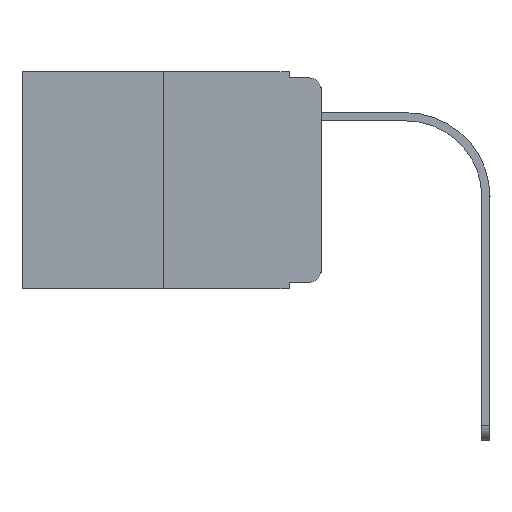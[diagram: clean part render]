
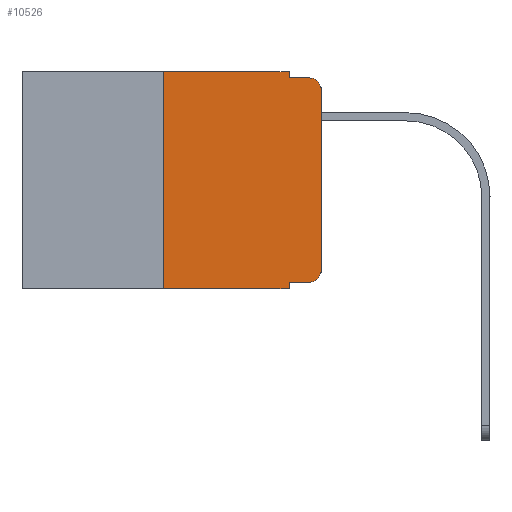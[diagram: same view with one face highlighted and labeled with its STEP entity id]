
A CAD part, left-side view. The second image highlights one B-rep face of the part: STEP entity #10526.
In plain terms, the highlighted planar face has unit normal (-1, 0, 0).
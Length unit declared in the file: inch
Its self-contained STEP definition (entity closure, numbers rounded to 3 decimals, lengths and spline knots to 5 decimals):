
#642 = ORIENTED_EDGE ( 'NONE', *, *, #10785, .F. ) ;
#699 = VERTEX_POINT ( 'NONE', #12797 ) ;
#761 = ORIENTED_EDGE ( 'NONE', *, *, #13675, .T. ) ;
#852 = LINE ( 'NONE', #12098, #2911 ) ;
#1095 = DIRECTION ( 'NONE',  ( 0., 0., -1. ) ) ;
#1178 = DIRECTION ( 'NONE',  ( 1., 0., 0. ) ) ;
#1365 = VERTEX_POINT ( 'NONE', #4801 ) ;
#1489 = DIRECTION ( 'NONE',  ( -1., 0., 0. ) ) ;
#1663 = VECTOR ( 'NONE', #3210, 39.37008 ) ;
#1671 = ORIENTED_EDGE ( 'NONE', *, *, #2084, .F. ) ;
#1684 = DIRECTION ( 'NONE',  ( -1., 0., 0. ) ) ;
#1687 = VECTOR ( 'NONE', #1709, 39.37008 ) ;
#1709 = DIRECTION ( 'NONE',  ( 0., -1., 0. ) ) ;
#1920 = CARTESIAN_POINT ( 'NONE',  ( 0., 0.051, -0.333 ) ) ;
#1997 = CARTESIAN_POINT ( 'NONE',  ( 0., 0.02, -0.333 ) ) ;
#2084 = EDGE_CURVE ( 'NONE', #699, #5482, #10360, .T. ) ;
#2117 = VECTOR ( 'NONE', #14281, 39.37008 ) ;
#2717 = LINE ( 'NONE', #15356, #7923 ) ;
#2911 = VECTOR ( 'NONE', #8301, 39.37008 ) ;
#3184 = VECTOR ( 'NONE', #4369, 39.37008 ) ;
#3191 = EDGE_CURVE ( 'NONE', #8622, #5011, #15493, .T. ) ;
#3210 = DIRECTION ( 'NONE',  ( 0., -1., 0. ) ) ;
#3257 = ORIENTED_EDGE ( 'NONE', *, *, #3451, .F. ) ;
#3451 = EDGE_CURVE ( 'NONE', #8622, #6676, #2717, .T. ) ;
#3988 = AXIS2_PLACEMENT_3D ( 'NONE', #4334, #1684, #9280 ) ;
#4334 = CARTESIAN_POINT ( 'NONE',  ( 0., 0.02, -0.03 ) ) ;
#4351 = EDGE_CURVE ( 'NONE', #5482, #6927, #13937, .T. ) ;
#4356 = CARTESIAN_POINT ( 'NONE',  ( 0., 0., -0.03 ) ) ;
#4369 = DIRECTION ( 'NONE',  ( 0., 0., -1. ) ) ;
#4468 = ORIENTED_EDGE ( 'NONE', *, *, #3191, .T. ) ;
#4512 = EDGE_CURVE ( 'NONE', #13848, #5011, #5578, .T. ) ;
#4595 = CARTESIAN_POINT ( 'NONE',  ( 0., 0.25, -0.343 ) ) ;
#4801 = CARTESIAN_POINT ( 'NONE',  ( 0., 0., -0.313 ) ) ;
#5011 = VERTEX_POINT ( 'NONE', #14778 ) ;
#5345 = CARTESIAN_POINT ( 'NONE',  ( 0., 0.25, 0. ) ) ;
#5482 = VERTEX_POINT ( 'NONE', #10277 ) ;
#5578 = LINE ( 'NONE', #9300, #10788 ) ;
#5629 = LINE ( 'NONE', #1920, #1663 ) ;
#5694 = CARTESIAN_POINT ( 'NONE',  ( 0., 0.473, 0. ) ) ;
#6269 = PLANE ( 'NONE',  #9319 ) ;
#6667 = DIRECTION ( 'NONE',  ( 0., 0., 1. ) ) ;
#6676 = VERTEX_POINT ( 'NONE', #5345 ) ;
#6927 = VERTEX_POINT ( 'NONE', #15793 ) ;
#7727 = CIRCLE ( 'NONE', #10307, 0.02 ) ;
#7923 = VECTOR ( 'NONE', #6667, 39.37008 ) ;
#8301 = DIRECTION ( 'NONE',  ( 0., 0., 1. ) ) ;
#8622 = VERTEX_POINT ( 'NONE', #4595 ) ;
#8678 = VERTEX_POINT ( 'NONE', #4356 ) ;
#8835 = CARTESIAN_POINT ( 'NONE',  ( 0., 0.051, -0.01 ) ) ;
#8904 = CIRCLE ( 'NONE', #3988, 0.02 ) ;
#9280 = DIRECTION ( 'NONE',  ( 0., 0., -1. ) ) ;
#9300 = CARTESIAN_POINT ( 'NONE',  ( 0., 0.051, 0. ) ) ;
#9319 = AXIS2_PLACEMENT_3D ( 'NONE', #16005, #1178, #1095 ) ;
#9321 = CARTESIAN_POINT ( 'NONE',  ( 0., 0.473, -0.343 ) ) ;
#9841 = VECTOR ( 'NONE', #15437, 39.37008 ) ;
#10277 = CARTESIAN_POINT ( 'NONE',  ( 0., 0.051, -0.01 ) ) ;
#10307 = AXIS2_PLACEMENT_3D ( 'NONE', #12580, #1489, #14788 ) ;
#10360 = LINE ( 'NONE', #15482, #3184 ) ;
#10417 = VERTEX_POINT ( 'NONE', #1997 ) ;
#10526 = ADVANCED_FACE ( 'NONE', ( #11037 ), #6269, .F. ) ;
#10567 = EDGE_LOOP ( 'NONE', ( #11794, #761, #13533, #1671, #642, #3257, #4468, #12792, #12236, #14541 ) ) ;
#10785 = EDGE_CURVE ( 'NONE', #6676, #699, #12900, .T. ) ;
#10788 = VECTOR ( 'NONE', #11646, 39.37008 ) ;
#11037 = FACE_OUTER_BOUND ( 'NONE', #10567, .T. ) ;
#11646 = DIRECTION ( 'NONE',  ( 0., 0., -1. ) ) ;
#11794 = ORIENTED_EDGE ( 'NONE', *, *, #12463, .T. ) ;
#12098 = CARTESIAN_POINT ( 'NONE',  ( 0., 0., 0. ) ) ;
#12236 = ORIENTED_EDGE ( 'NONE', *, *, #13638, .T. ) ;
#12463 = EDGE_CURVE ( 'NONE', #1365, #8678, #852, .T. ) ;
#12580 = CARTESIAN_POINT ( 'NONE',  ( 0., 0.02, -0.313 ) ) ;
#12792 = ORIENTED_EDGE ( 'NONE', *, *, #4512, .F. ) ;
#12797 = CARTESIAN_POINT ( 'NONE',  ( 0., 0.051, 0. ) ) ;
#12900 = LINE ( 'NONE', #5694, #9841 ) ;
#13533 = ORIENTED_EDGE ( 'NONE', *, *, #4351, .F. ) ;
#13638 = EDGE_CURVE ( 'NONE', #13848, #10417, #5629, .T. ) ;
#13675 = EDGE_CURVE ( 'NONE', #8678, #6927, #8904, .T. ) ;
#13848 = VERTEX_POINT ( 'NONE', #16002 ) ;
#13937 = LINE ( 'NONE', #8835, #1687 ) ;
#14281 = DIRECTION ( 'NONE',  ( 0., -1., 0. ) ) ;
#14541 = ORIENTED_EDGE ( 'NONE', *, *, #15978, .T. ) ;
#14778 = CARTESIAN_POINT ( 'NONE',  ( 0., 0.051, -0.343 ) ) ;
#14788 = DIRECTION ( 'NONE',  ( 0., 0., -1. ) ) ;
#15356 = CARTESIAN_POINT ( 'NONE',  ( 0., 0.25, 0. ) ) ;
#15437 = DIRECTION ( 'NONE',  ( 0., -1., 0. ) ) ;
#15482 = CARTESIAN_POINT ( 'NONE',  ( 0., 0.051, 0. ) ) ;
#15493 = LINE ( 'NONE', #9321, #2117 ) ;
#15793 = CARTESIAN_POINT ( 'NONE',  ( 0., 0.02, -0.01 ) ) ;
#15978 = EDGE_CURVE ( 'NONE', #10417, #1365, #7727, .T. ) ;
#16002 = CARTESIAN_POINT ( 'NONE',  ( 0., 0.051, -0.333 ) ) ;
#16005 = CARTESIAN_POINT ( 'NONE',  ( 0., 0.473, 0. ) ) ;
